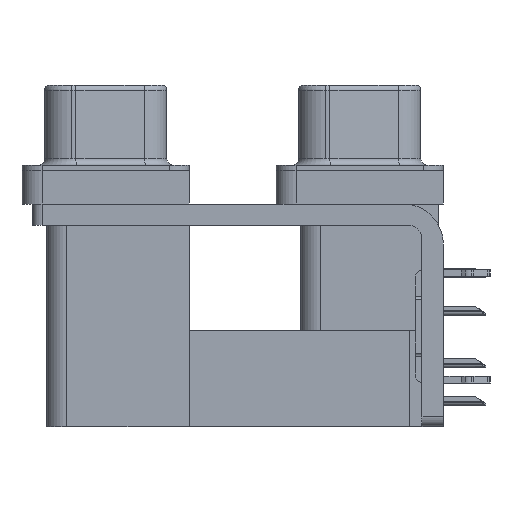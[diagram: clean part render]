
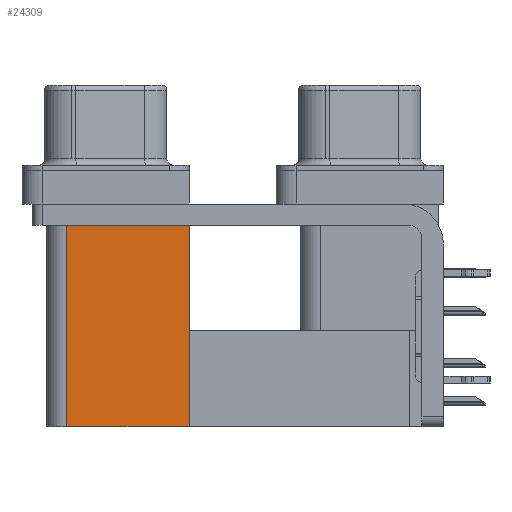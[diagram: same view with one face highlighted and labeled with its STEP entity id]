
A CAD part, left-side view. The second image highlights one B-rep face of the part: STEP entity #24309.
In plain terms, the highlighted planar face has unit normal (-1, 0, 0).
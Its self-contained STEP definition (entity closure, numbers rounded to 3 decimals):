
#2618 = DIRECTION ( 'NONE',  ( 0., 0., 1. ) ) ;
#3151 = PLANE ( 'NONE',  #22888 ) ;
#3593 = CARTESIAN_POINT ( 'NONE',  ( 3.7, 21.975, -2.5 ) ) ;
#4660 = EDGE_LOOP ( 'NONE', ( #33982, #38714, #35477, #11982 ) ) ;
#5214 = CARTESIAN_POINT ( 'NONE',  ( 3.7, 12.775, -19.2 ) ) ;
#5364 = LINE ( 'NONE', #24420, #18201 ) ;
#5717 = EDGE_CURVE ( 'NONE', #17565, #39791, #29721, .T. ) ;
#6537 = CARTESIAN_POINT ( 'NONE',  ( 3.7, 12.775, -19.2 ) ) ;
#8387 = CARTESIAN_POINT ( 'NONE',  ( 3.7, 12.775, -19.2 ) ) ;
#8414 = LINE ( 'NONE', #20918, #21072 ) ;
#9925 = CARTESIAN_POINT ( 'NONE',  ( 3.7, 12.775, -19.2 ) ) ;
#11105 = CARTESIAN_POINT ( 'NONE',  ( 3.7, 21.975, -19.2 ) ) ;
#11982 = ORIENTED_EDGE ( 'NONE', *, *, #12380, .T. ) ;
#12380 = EDGE_CURVE ( 'NONE', #17565, #25563, #24557, .T. ) ;
#14376 = DIRECTION ( 'NONE',  ( 0., 0., 1. ) ) ;
#17318 = VERTEX_POINT ( 'NONE', #3593 ) ;
#17565 = VERTEX_POINT ( 'NONE', #5214 ) ;
#17890 = VECTOR ( 'NONE', #2618, 1000. ) ;
#18201 = VECTOR ( 'NONE', #30003, 1000. ) ;
#20918 = CARTESIAN_POINT ( 'NONE',  ( 3.7, 21.975, -19.2 ) ) ;
#21072 = VECTOR ( 'NONE', #14376, 1000. ) ;
#22149 = EDGE_CURVE ( 'NONE', #25563, #17318, #5364, .T. ) ;
#22888 = AXIS2_PLACEMENT_3D ( 'NONE', #9925, #24882, #40454 ) ;
#23738 = DIRECTION ( 'NONE',  ( 0., 1., 0. ) ) ;
#24309 = ADVANCED_FACE ( 'NONE', ( #38184 ), #3151, .F. ) ;
#24420 = CARTESIAN_POINT ( 'NONE',  ( 3.7, 12.775, -2.5 ) ) ;
#24557 = LINE ( 'NONE', #6537, #17890 ) ;
#24882 = DIRECTION ( 'NONE',  ( 1., 0., 0. ) ) ;
#25563 = VERTEX_POINT ( 'NONE', #37032 ) ;
#29103 = VECTOR ( 'NONE', #23738, 1000. ) ;
#29721 = LINE ( 'NONE', #8387, #29103 ) ;
#30003 = DIRECTION ( 'NONE',  ( 0., 1., 0. ) ) ;
#33982 = ORIENTED_EDGE ( 'NONE', *, *, #22149, .T. ) ;
#35477 = ORIENTED_EDGE ( 'NONE', *, *, #5717, .F. ) ;
#37032 = CARTESIAN_POINT ( 'NONE',  ( 3.7, 12.775, -2.5 ) ) ;
#38184 = FACE_OUTER_BOUND ( 'NONE', #4660, .T. ) ;
#38630 = EDGE_CURVE ( 'NONE', #39791, #17318, #8414, .T. ) ;
#38714 = ORIENTED_EDGE ( 'NONE', *, *, #38630, .F. ) ;
#39791 = VERTEX_POINT ( 'NONE', #11105 ) ;
#40454 = DIRECTION ( 'NONE',  ( 0., 1., 0. ) ) ;
